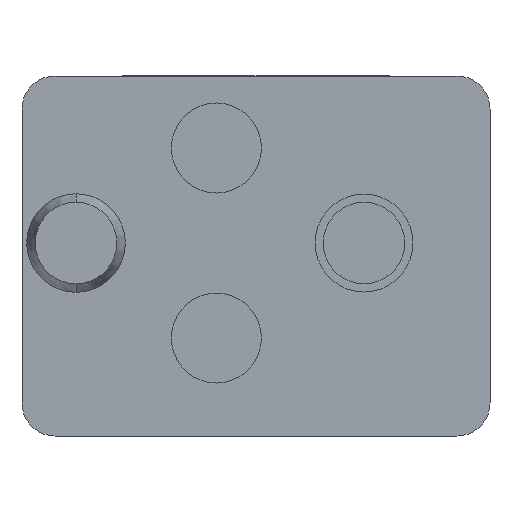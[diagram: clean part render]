
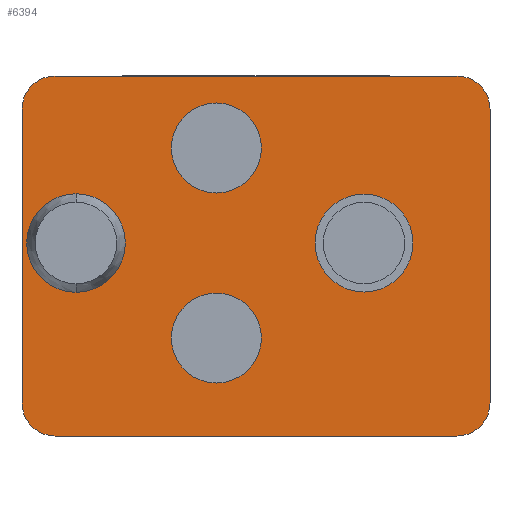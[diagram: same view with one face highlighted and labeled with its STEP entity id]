
A CAD part, front view. The second image highlights one B-rep face of the part: STEP entity #6394.
In plain terms, the highlighted planar face has unit normal (0, -1, 0).
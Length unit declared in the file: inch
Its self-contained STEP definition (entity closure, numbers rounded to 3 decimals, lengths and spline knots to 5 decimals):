
#56 = VERTEX_POINT ( 'NONE', #1934 ) ;
#61 = EDGE_CURVE ( 'NONE', #2830, #6130, #2871, .T. ) ;
#110 = EDGE_LOOP ( 'NONE', ( #1412, #3274, #1722, #3382, #6174, #1298, #3126, #831 ) ) ;
#205 = CARTESIAN_POINT ( 'NONE',  ( -0.325, 0., 0.204 ) ) ;
#207 = DIRECTION ( 'NONE',  ( 1., 0., 0. ) ) ;
#303 = EDGE_LOOP ( 'NONE', ( #1429, #2634 ) ) ;
#308 = EDGE_CURVE ( 'NONE', #5235, #2716, #2004, .T. ) ;
#355 = DIRECTION ( 'NONE',  ( 0., 0., -1. ) ) ;
#358 = DIRECTION ( 'NONE',  ( -1., 0., 0. ) ) ;
#386 = EDGE_CURVE ( 'NONE', #2491, #1984, #492, .T. ) ;
#412 = CARTESIAN_POINT ( 'NONE',  ( 0.325, 0., 0.204 ) ) ;
#481 = CARTESIAN_POINT ( 'NONE',  ( -0.325, 0., -0.204 ) ) ;
#492 = CIRCLE ( 'NONE', #1424, 0.068 ) ;
#584 = DIRECTION ( 'NONE',  ( 0., 0., -1. ) ) ;
#662 = CARTESIAN_POINT ( 'NONE',  ( 0.279, 0., 0.204 ) ) ;
#755 = DIRECTION ( 'NONE',  ( 0., 0., -1. ) ) ;
#783 = EDGE_CURVE ( 'NONE', #2050, #3536, #5323, .T. ) ;
#795 = VERTEX_POINT ( 'NONE', #4203 ) ;
#810 = CARTESIAN_POINT ( 'NONE',  ( 0.15, 0., 0.018 ) ) ;
#831 = ORIENTED_EDGE ( 'NONE', *, *, #5984, .F. ) ;
#832 = EDGE_LOOP ( 'NONE', ( #871, #6080 ) ) ;
#871 = ORIENTED_EDGE ( 'NONE', *, *, #6674, .F. ) ;
#953 = DIRECTION ( 'NONE',  ( 0., 0., -1. ) ) ;
#1002 = FACE_BOUND ( 'NONE', #832, .T. ) ;
#1077 = FACE_BOUND ( 'NONE', #2627, .T. ) ;
#1183 = AXIS2_PLACEMENT_3D ( 'NONE', #4213, #1452, #1415 ) ;
#1298 = ORIENTED_EDGE ( 'NONE', *, *, #2094, .F. ) ;
#1305 = CIRCLE ( 'NONE', #5676, 0.0625 ) ;
#1412 = ORIENTED_EDGE ( 'NONE', *, *, #783, .F. ) ;
#1415 = DIRECTION ( 'NONE',  ( 0., 0., -1. ) ) ;
#1424 = AXIS2_PLACEMENT_3D ( 'NONE', #2856, #5399, #355 ) ;
#1429 = ORIENTED_EDGE ( 'NONE', *, *, #3501, .F. ) ;
#1452 = DIRECTION ( 'NONE',  ( 0., -1., 0. ) ) ;
#1527 = AXIS2_PLACEMENT_3D ( 'NONE', #4129, #4202, #4688 ) ;
#1551 = FACE_BOUND ( 'NONE', #1883, .T. ) ;
#1557 = DIRECTION ( 'NONE',  ( 0., 0., -1. ) ) ;
#1722 = ORIENTED_EDGE ( 'NONE', *, *, #308, .F. ) ;
#1852 = EDGE_CURVE ( 'NONE', #5952, #2857, #6716, .T. ) ;
#1855 = DIRECTION ( 'NONE',  ( 0., 0., 1. ) ) ;
#1875 = VERTEX_POINT ( 'NONE', #6140 ) ;
#1883 = EDGE_LOOP ( 'NONE', ( #6868, #7140 ) ) ;
#1891 = CARTESIAN_POINT ( 'NONE',  ( -0.325, 0., 0.204 ) ) ;
#1934 = CARTESIAN_POINT ( 'NONE',  ( -0.055, 0., 0.2125 ) ) ;
#1984 = VERTEX_POINT ( 'NONE', #2745 ) ;
#2004 = CIRCLE ( 'NONE', #6500, 0.046 ) ;
#2030 = CARTESIAN_POINT ( 'NONE',  ( -0.279, 0., -0.204 ) ) ;
#2037 = CARTESIAN_POINT ( 'NONE',  ( -0.279, 0., -0.25 ) ) ;
#2050 = VERTEX_POINT ( 'NONE', #3070 ) ;
#2067 = VECTOR ( 'NONE', #207, 39.37008 ) ;
#2094 = EDGE_CURVE ( 'NONE', #2857, #5091, #3670, .T. ) ;
#2133 = AXIS2_PLACEMENT_3D ( 'NONE', #2501, #5873, #755 ) ;
#2244 = VECTOR ( 'NONE', #4926, 39.37008 ) ;
#2307 = CIRCLE ( 'NONE', #6448, 0.0625 ) ;
#2475 = CARTESIAN_POINT ( 'NONE',  ( 0.279, 0., -0.25 ) ) ;
#2491 = VERTEX_POINT ( 'NONE', #6802 ) ;
#2501 = CARTESIAN_POINT ( 'NONE',  ( 0.279, 0., -0.204 ) ) ;
#2540 = DIRECTION ( 'NONE',  ( 0., -1., 0. ) ) ;
#2627 = EDGE_LOOP ( 'NONE', ( #6505, #4954 ) ) ;
#2634 = ORIENTED_EDGE ( 'NONE', *, *, #61, .F. ) ;
#2716 = VERTEX_POINT ( 'NONE', #412 ) ;
#2745 = CARTESIAN_POINT ( 'NONE',  ( 0.15, 0., 0.086 ) ) ;
#2788 = DIRECTION ( 'NONE',  ( 0., 0., -1. ) ) ;
#2830 = VERTEX_POINT ( 'NONE', #3384 ) ;
#2856 = CARTESIAN_POINT ( 'NONE',  ( 0.15, 0., 0.018 ) ) ;
#2857 = VERTEX_POINT ( 'NONE', #481 ) ;
#2871 = CIRCLE ( 'NONE', #3812, 0.0685 ) ;
#3070 = CARTESIAN_POINT ( 'NONE',  ( 0.325, 0., -0.204 ) ) ;
#3102 = DIRECTION ( 'NONE',  ( 0., 1., 0. ) ) ;
#3126 = ORIENTED_EDGE ( 'NONE', *, *, #1852, .F. ) ;
#3179 = CARTESIAN_POINT ( 'NONE',  ( -0.279, 0., -0.25 ) ) ;
#3205 = FACE_BOUND ( 'NONE', #303, .T. ) ;
#3221 = EDGE_CURVE ( 'NONE', #5091, #795, #5096, .T. ) ;
#3274 = ORIENTED_EDGE ( 'NONE', *, *, #3982, .F. ) ;
#3292 = CIRCLE ( 'NONE', #1527, 0.0625 ) ;
#3342 = DIRECTION ( 'NONE',  ( 0., 1., 0. ) ) ;
#3382 = ORIENTED_EDGE ( 'NONE', *, *, #5808, .F. ) ;
#3384 = CARTESIAN_POINT ( 'NONE',  ( -0.25, 0., -0.0505 ) ) ;
#3423 = CARTESIAN_POINT ( 'NONE',  ( -0.055, 0., -0.1765 ) ) ;
#3501 = EDGE_CURVE ( 'NONE', #6130, #2830, #5181, .T. ) ;
#3527 = DIRECTION ( 'NONE',  ( 0., 0., -1. ) ) ;
#3536 = VERTEX_POINT ( 'NONE', #2475 ) ;
#3670 = LINE ( 'NONE', #1891, #6968 ) ;
#3744 = DIRECTION ( 'NONE',  ( 0., -1., 0. ) ) ;
#3792 = DIRECTION ( 'NONE',  ( 0., -1., 0. ) ) ;
#3801 = FACE_OUTER_BOUND ( 'NONE', #110, .T. ) ;
#3812 = AXIS2_PLACEMENT_3D ( 'NONE', #4713, #4189, #3527 ) ;
#3864 = EDGE_CURVE ( 'NONE', #56, #1875, #3292, .T. ) ;
#3982 = EDGE_CURVE ( 'NONE', #2716, #2050, #4963, .T. ) ;
#4129 = CARTESIAN_POINT ( 'NONE',  ( -0.055, 0., 0.15 ) ) ;
#4189 = DIRECTION ( 'NONE',  ( 0., -1., 0. ) ) ;
#4202 = DIRECTION ( 'NONE',  ( 0., -1., 0. ) ) ;
#4203 = CARTESIAN_POINT ( 'NONE',  ( -0.279, 0., 0.25 ) ) ;
#4213 = CARTESIAN_POINT ( 'NONE',  ( -0.25, 0., 0.018 ) ) ;
#4262 = EDGE_CURVE ( 'NONE', #1875, #56, #1305, .T. ) ;
#4321 = DIRECTION ( 'NONE',  ( 0., -1., 0. ) ) ;
#4326 = AXIS2_PLACEMENT_3D ( 'NONE', #810, #3744, #953 ) ;
#4372 = CARTESIAN_POINT ( 'NONE',  ( -0.279, 0., 0.204 ) ) ;
#4410 = DIRECTION ( 'NONE',  ( 0., 1., 0. ) ) ;
#4431 = PLANE ( 'NONE',  #5490 ) ;
#4476 = CARTESIAN_POINT ( 'NONE',  ( 0.279, 0., 0.25 ) ) ;
#4504 = AXIS2_PLACEMENT_3D ( 'NONE', #4372, #4410, #584 ) ;
#4688 = DIRECTION ( 'NONE',  ( 0., 0., -1. ) ) ;
#4713 = CARTESIAN_POINT ( 'NONE',  ( -0.25, 0., 0.018 ) ) ;
#4721 = EDGE_CURVE ( 'NONE', #7203, #5597, #2307, .T. ) ;
#4805 = DIRECTION ( 'NONE',  ( 0., 0., -1. ) ) ;
#4904 = AXIS2_PLACEMENT_3D ( 'NONE', #6423, #6347, #6460 ) ;
#4926 = DIRECTION ( 'NONE',  ( 0., 0., -1. ) ) ;
#4954 = ORIENTED_EDGE ( 'NONE', *, *, #3864, .F. ) ;
#4963 = LINE ( 'NONE', #5515, #2244 ) ;
#5091 = VERTEX_POINT ( 'NONE', #205 ) ;
#5096 = CIRCLE ( 'NONE', #4504, 0.046 ) ;
#5181 = CIRCLE ( 'NONE', #1183, 0.0685 ) ;
#5235 = VERTEX_POINT ( 'NONE', #4476 ) ;
#5251 = CARTESIAN_POINT ( 'NONE',  ( -0.279, 0., 0.25 ) ) ;
#5323 = CIRCLE ( 'NONE', #2133, 0.046 ) ;
#5399 = DIRECTION ( 'NONE',  ( 0., -1., 0. ) ) ;
#5490 = AXIS2_PLACEMENT_3D ( 'NONE', #6061, #4321, #7244 ) ;
#5515 = CARTESIAN_POINT ( 'NONE',  ( 0.325, 0., 0.204 ) ) ;
#5597 = VERTEX_POINT ( 'NONE', #3423 ) ;
#5615 = EDGE_CURVE ( 'NONE', #1984, #2491, #7281, .T. ) ;
#5676 = AXIS2_PLACEMENT_3D ( 'NONE', #6059, #2540, #4805 ) ;
#5808 = EDGE_CURVE ( 'NONE', #795, #5235, #6788, .T. ) ;
#5851 = LINE ( 'NONE', #2037, #5853 ) ;
#5853 = VECTOR ( 'NONE', #358, 39.37008 ) ;
#5873 = DIRECTION ( 'NONE',  ( 0., 1., 0. ) ) ;
#5952 = VERTEX_POINT ( 'NONE', #3179 ) ;
#5984 = EDGE_CURVE ( 'NONE', #3536, #5952, #5851, .T. ) ;
#6059 = CARTESIAN_POINT ( 'NONE',  ( -0.055, 0., 0.15 ) ) ;
#6061 = CARTESIAN_POINT ( 'NONE',  ( 0.279, 0., -0.204 ) ) ;
#6080 = ORIENTED_EDGE ( 'NONE', *, *, #4721, .F. ) ;
#6115 = AXIS2_PLACEMENT_3D ( 'NONE', #2030, #3102, #1557 ) ;
#6130 = VERTEX_POINT ( 'NONE', #6635 ) ;
#6140 = CARTESIAN_POINT ( 'NONE',  ( -0.055, 0., 0.0875 ) ) ;
#6174 = ORIENTED_EDGE ( 'NONE', *, *, #3221, .F. ) ;
#6190 = DIRECTION ( 'NONE',  ( 0., 0., 1. ) ) ;
#6347 = DIRECTION ( 'NONE',  ( 0., -1., 0. ) ) ;
#6394 = ADVANCED_FACE ( 'NONE', ( #1551, #1002, #1077, #3205, #3801 ), #4431, .T. ) ;
#6423 = CARTESIAN_POINT ( 'NONE',  ( -0.055, 0., -0.114 ) ) ;
#6448 = AXIS2_PLACEMENT_3D ( 'NONE', #6683, #3792, #2788 ) ;
#6460 = DIRECTION ( 'NONE',  ( 0., 0., -1. ) ) ;
#6500 = AXIS2_PLACEMENT_3D ( 'NONE', #662, #3342, #6190 ) ;
#6505 = ORIENTED_EDGE ( 'NONE', *, *, #4262, .F. ) ;
#6635 = CARTESIAN_POINT ( 'NONE',  ( -0.25, 0., 0.0865 ) ) ;
#6674 = EDGE_CURVE ( 'NONE', #5597, #7203, #7152, .T. ) ;
#6683 = CARTESIAN_POINT ( 'NONE',  ( -0.055, 0., -0.114 ) ) ;
#6716 = CIRCLE ( 'NONE', #6115, 0.046 ) ;
#6788 = LINE ( 'NONE', #5251, #2067 ) ;
#6802 = CARTESIAN_POINT ( 'NONE',  ( 0.15, 0., -0.05 ) ) ;
#6868 = ORIENTED_EDGE ( 'NONE', *, *, #386, .F. ) ;
#6878 = CARTESIAN_POINT ( 'NONE',  ( -0.055, 0., -0.0515 ) ) ;
#6968 = VECTOR ( 'NONE', #1855, 39.37008 ) ;
#7140 = ORIENTED_EDGE ( 'NONE', *, *, #5615, .F. ) ;
#7152 = CIRCLE ( 'NONE', #4904, 0.0625 ) ;
#7203 = VERTEX_POINT ( 'NONE', #6878 ) ;
#7244 = DIRECTION ( 'NONE',  ( 0., 0., -1. ) ) ;
#7281 = CIRCLE ( 'NONE', #4326, 0.068 ) ;
